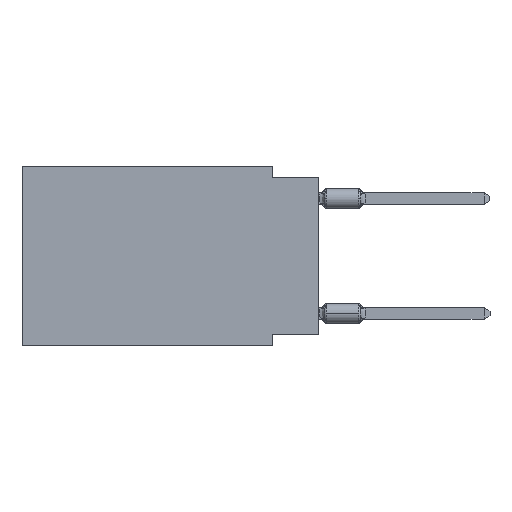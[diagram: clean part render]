
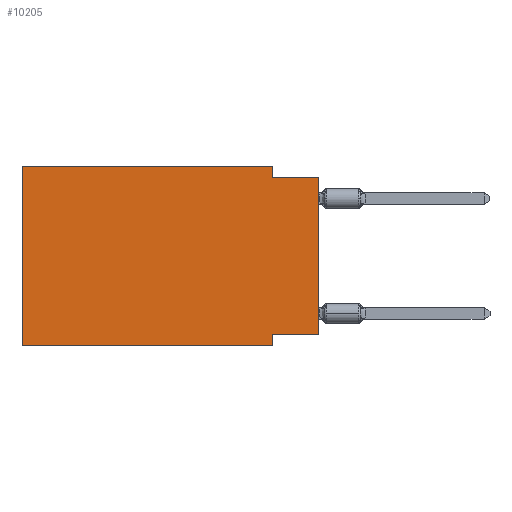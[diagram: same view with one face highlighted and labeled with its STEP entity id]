
A CAD part, left-side view. The second image highlights one B-rep face of the part: STEP entity #10205.
In plain terms, the highlighted planar face has unit normal (-1, 0, 0).
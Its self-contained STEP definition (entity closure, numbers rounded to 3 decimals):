
#54 = DIRECTION ( 'NONE',  ( 0., -1., 0. ) ) ;
#102 = DIRECTION ( 'NONE',  ( 0., -1., 0. ) ) ;
#661 = CARTESIAN_POINT ( 'NONE',  ( 0., 16.383, 0. ) ) ;
#1351 = EDGE_CURVE ( 'NONE', #15175, #11374, #4896, .T. ) ;
#1604 = VERTEX_POINT ( 'NONE', #19011 ) ;
#1831 = LINE ( 'NONE', #19329, #4510 ) ;
#2209 = VERTEX_POINT ( 'NONE', #20952 ) ;
#2698 = ORIENTED_EDGE ( 'NONE', *, *, #11360, .T. ) ;
#3220 = DIRECTION ( 'NONE',  ( 0., 1., 0. ) ) ;
#3253 = EDGE_CURVE ( 'NONE', #1604, #9902, #13527, .T. ) ;
#3795 = DIRECTION ( 'NONE',  ( 0., -1., 0. ) ) ;
#4010 = VERTEX_POINT ( 'NONE', #21891 ) ;
#4082 = VERTEX_POINT ( 'NONE', #6915 ) ;
#4132 = CARTESIAN_POINT ( 'NONE',  ( 0., 2.54, -9.271 ) ) ;
#4195 = CARTESIAN_POINT ( 'NONE',  ( 0., 16.383, 0. ) ) ;
#4510 = VECTOR ( 'NONE', #3220, 1000. ) ;
#4517 = PLANE ( 'NONE',  #13554 ) ;
#4784 = DIRECTION ( 'NONE',  ( 0., 0., 1. ) ) ;
#4896 = LINE ( 'NONE', #14179, #7815 ) ;
#5519 = LINE ( 'NONE', #10619, #19704 ) ;
#5622 = VECTOR ( 'NONE', #102, 1000. ) ;
#6915 = CARTESIAN_POINT ( 'NONE',  ( 0., 16.383, -9.906 ) ) ;
#6960 = ORIENTED_EDGE ( 'NONE', *, *, #15004, .F. ) ;
#7815 = VECTOR ( 'NONE', #17113, 1000. ) ;
#7897 = LINE ( 'NONE', #11592, #21269 ) ;
#9604 = LINE ( 'NONE', #4195, #12999 ) ;
#9854 = EDGE_CURVE ( 'NONE', #20401, #4010, #7897, .T. ) ;
#9902 = VERTEX_POINT ( 'NONE', #19874 ) ;
#10205 = ADVANCED_FACE ( 'NONE', ( #20289 ), #4517, .F. ) ;
#10373 = ORIENTED_EDGE ( 'NONE', *, *, #3253, .T. ) ;
#10619 = CARTESIAN_POINT ( 'NONE',  ( 0., 16.383, -9.906 ) ) ;
#11177 = VECTOR ( 'NONE', #4784, 1000. ) ;
#11360 = EDGE_CURVE ( 'NONE', #4082, #4010, #5519, .T. ) ;
#11374 = VERTEX_POINT ( 'NONE', #18072 ) ;
#11556 = DIRECTION ( 'NONE',  ( 1., 0., 0. ) ) ;
#11592 = CARTESIAN_POINT ( 'NONE',  ( 0., 2.54, -9.906 ) ) ;
#11731 = ORIENTED_EDGE ( 'NONE', *, *, #9854, .F. ) ;
#12041 = ORIENTED_EDGE ( 'NONE', *, *, #13435, .F. ) ;
#12999 = VECTOR ( 'NONE', #14130, 1000. ) ;
#13081 = EDGE_LOOP ( 'NONE', ( #10373, #12041, #14825, #6960, #19293, #2698, #11731, #13120 ) ) ;
#13120 = ORIENTED_EDGE ( 'NONE', *, *, #20704, .F. ) ;
#13435 = EDGE_CURVE ( 'NONE', #11374, #9902, #19631, .T. ) ;
#13527 = LINE ( 'NONE', #20562, #11177 ) ;
#13554 = AXIS2_PLACEMENT_3D ( 'NONE', #18351, #11556, #18575 ) ;
#14130 = DIRECTION ( 'NONE',  ( 0., 0., 1. ) ) ;
#14179 = CARTESIAN_POINT ( 'NONE',  ( 0., 2.54, 0. ) ) ;
#14274 = CARTESIAN_POINT ( 'NONE',  ( 0., 2.54, 0. ) ) ;
#14825 = ORIENTED_EDGE ( 'NONE', *, *, #1351, .F. ) ;
#15004 = EDGE_CURVE ( 'NONE', #2209, #15175, #15879, .T. ) ;
#15175 = VERTEX_POINT ( 'NONE', #14274 ) ;
#15497 = EDGE_CURVE ( 'NONE', #4082, #2209, #9604, .T. ) ;
#15879 = LINE ( 'NONE', #661, #5622 ) ;
#17113 = DIRECTION ( 'NONE',  ( 0., 0., -1. ) ) ;
#17685 = CARTESIAN_POINT ( 'NONE',  ( 0., 0., -0.635 ) ) ;
#18072 = CARTESIAN_POINT ( 'NONE',  ( 0., 2.54, -0.635 ) ) ;
#18351 = CARTESIAN_POINT ( 'NONE',  ( 0., 16.383, 0. ) ) ;
#18575 = DIRECTION ( 'NONE',  ( 0., 0., -1. ) ) ;
#19011 = CARTESIAN_POINT ( 'NONE',  ( 0., 0., -9.271 ) ) ;
#19293 = ORIENTED_EDGE ( 'NONE', *, *, #15497, .F. ) ;
#19329 = CARTESIAN_POINT ( 'NONE',  ( 0., 0., -9.271 ) ) ;
#19631 = LINE ( 'NONE', #17685, #20841 ) ;
#19704 = VECTOR ( 'NONE', #3795, 1000. ) ;
#19874 = CARTESIAN_POINT ( 'NONE',  ( 0., 0., -0.635 ) ) ;
#19983 = DIRECTION ( 'NONE',  ( 0., 0., -1. ) ) ;
#20289 = FACE_OUTER_BOUND ( 'NONE', #13081, .T. ) ;
#20401 = VERTEX_POINT ( 'NONE', #4132 ) ;
#20562 = CARTESIAN_POINT ( 'NONE',  ( 0., 0., 0. ) ) ;
#20704 = EDGE_CURVE ( 'NONE', #1604, #20401, #1831, .T. ) ;
#20841 = VECTOR ( 'NONE', #54, 1000. ) ;
#20952 = CARTESIAN_POINT ( 'NONE',  ( 0., 16.383, 0. ) ) ;
#21269 = VECTOR ( 'NONE', #19983, 1000. ) ;
#21891 = CARTESIAN_POINT ( 'NONE',  ( 0., 2.54, -9.906 ) ) ;
